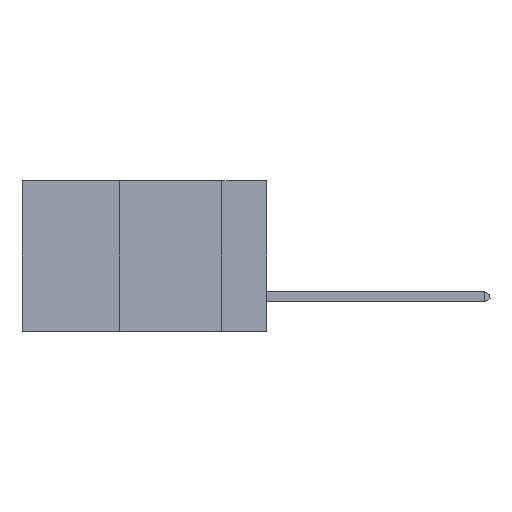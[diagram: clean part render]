
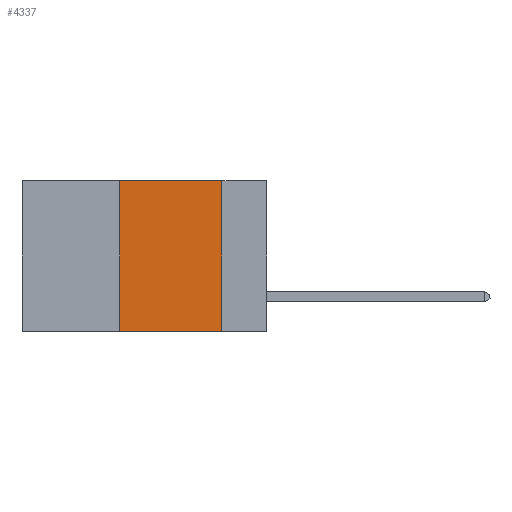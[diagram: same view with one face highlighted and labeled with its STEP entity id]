
A CAD part, left-side view. The second image highlights one B-rep face of the part: STEP entity #4337.
In plain terms, the highlighted planar face has unit normal (-1, 0, 0).
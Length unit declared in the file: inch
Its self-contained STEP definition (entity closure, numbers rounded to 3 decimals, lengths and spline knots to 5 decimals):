
#166 = DIRECTION ( 'NONE',  ( 0., 0., -1. ) ) ;
#1340 = LINE ( 'NONE', #21598, #10885 ) ;
#1420 = LINE ( 'NONE', #8237, #19338 ) ;
#1965 = EDGE_LOOP ( 'NONE', ( #12650, #5268, #16562, #19646 ) ) ;
#2335 = VECTOR ( 'NONE', #10147, 39.37008 ) ;
#2770 = AXIS2_PLACEMENT_3D ( 'NONE', #5073, #4920, #4891 ) ;
#3666 = VERTEX_POINT ( 'NONE', #16074 ) ;
#4337 = ADVANCED_FACE ( 'NONE', ( #10812 ), #4945, .F. ) ;
#4891 = DIRECTION ( 'NONE',  ( 0., 0., -1. ) ) ;
#4920 = DIRECTION ( 'NONE',  ( 1., 0., 0. ) ) ;
#4945 = PLANE ( 'NONE',  #2770 ) ;
#5073 = CARTESIAN_POINT ( 'NONE',  ( 0., 0.6, 0. ) ) ;
#5242 = CARTESIAN_POINT ( 'NONE',  ( 0., 0.6, 0. ) ) ;
#5268 = ORIENTED_EDGE ( 'NONE', *, *, #17627, .F. ) ;
#5681 = CARTESIAN_POINT ( 'NONE',  ( 0., 0.11, -0.37 ) ) ;
#8237 = CARTESIAN_POINT ( 'NONE',  ( 0., 0.36, 0. ) ) ;
#8354 = CARTESIAN_POINT ( 'NONE',  ( 0., 0.6, -0.37 ) ) ;
#10147 = DIRECTION ( 'NONE',  ( 0., -1., 0. ) ) ;
#10812 = FACE_OUTER_BOUND ( 'NONE', #1965, .T. ) ;
#10885 = VECTOR ( 'NONE', #166, 39.37008 ) ;
#12650 = ORIENTED_EDGE ( 'NONE', *, *, #18386, .F. ) ;
#13117 = VERTEX_POINT ( 'NONE', #14861 ) ;
#14583 = LINE ( 'NONE', #5242, #18214 ) ;
#14861 = CARTESIAN_POINT ( 'NONE',  ( 0., 0.36, -0.37 ) ) ;
#15351 = CARTESIAN_POINT ( 'NONE',  ( 0., 0.36, 0. ) ) ;
#16074 = CARTESIAN_POINT ( 'NONE',  ( 0., 0.11, 0. ) ) ;
#16559 = VERTEX_POINT ( 'NONE', #5681 ) ;
#16562 = ORIENTED_EDGE ( 'NONE', *, *, #23008, .F. ) ;
#16631 = LINE ( 'NONE', #8354, #2335 ) ;
#17184 = DIRECTION ( 'NONE',  ( 0., 0., 1. ) ) ;
#17627 = EDGE_CURVE ( 'NONE', #21357, #3666, #14583, .T. ) ;
#17774 = DIRECTION ( 'NONE',  ( 0., -1., 0. ) ) ;
#18214 = VECTOR ( 'NONE', #17774, 39.37008 ) ;
#18386 = EDGE_CURVE ( 'NONE', #3666, #16559, #1340, .T. ) ;
#19338 = VECTOR ( 'NONE', #17184, 39.37008 ) ;
#19646 = ORIENTED_EDGE ( 'NONE', *, *, #21862, .T. ) ;
#21357 = VERTEX_POINT ( 'NONE', #15351 ) ;
#21598 = CARTESIAN_POINT ( 'NONE',  ( 0., 0.11, 0. ) ) ;
#21862 = EDGE_CURVE ( 'NONE', #13117, #16559, #16631, .T. ) ;
#23008 = EDGE_CURVE ( 'NONE', #13117, #21357, #1420, .T. ) ;
